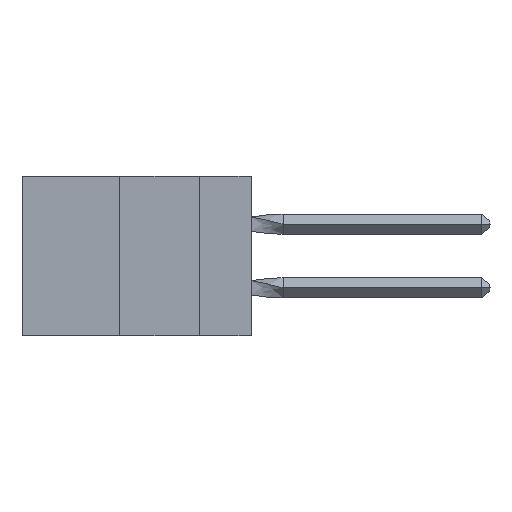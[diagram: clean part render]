
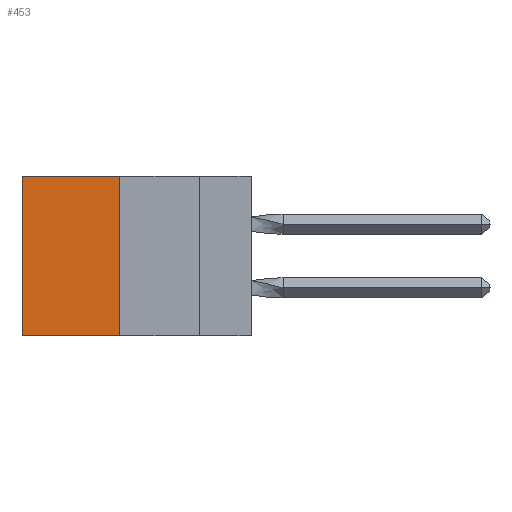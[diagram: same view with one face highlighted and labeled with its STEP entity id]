
A CAD part, left-side view. The second image highlights one B-rep face of the part: STEP entity #453.
In plain terms, the highlighted planar face has unit normal (-1, 0, 0).
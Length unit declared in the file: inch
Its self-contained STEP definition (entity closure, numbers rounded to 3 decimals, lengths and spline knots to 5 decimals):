
#450 = EDGE_CURVE ( 'NONE', #2430, #16674, #26273, .T. ) ;
#453 = ADVANCED_FACE ( 'NONE', ( #7988 ), #14842, .F. ) ;
#598 = EDGE_CURVE ( 'NONE', #6258, #15881, #14458, .T. ) ;
#779 = LINE ( 'NONE', #3295, #23104 ) ;
#1142 = CARTESIAN_POINT ( 'NONE',  ( 0.305, 0.72, 0. ) ) ;
#2425 = DIRECTION ( 'NONE',  ( 0., 0., -1. ) ) ;
#2430 = VERTEX_POINT ( 'NONE', #19436 ) ;
#3295 = CARTESIAN_POINT ( 'NONE',  ( 0.305, 0.413, 0. ) ) ;
#5922 = ORIENTED_EDGE ( 'NONE', *, *, #598, .T. ) ;
#6258 = VERTEX_POINT ( 'NONE', #1142 ) ;
#6452 = EDGE_CURVE ( 'NONE', #16674, #15881, #7986, .T. ) ;
#6819 = CARTESIAN_POINT ( 'NONE',  ( 0.305, 0.72, -0.5 ) ) ;
#7986 = LINE ( 'NONE', #21647, #10041 ) ;
#7988 = FACE_OUTER_BOUND ( 'NONE', #17832, .T. ) ;
#8492 = ORIENTED_EDGE ( 'NONE', *, *, #6452, .F. ) ;
#8943 = DIRECTION ( 'NONE',  ( 0., 1., 0. ) ) ;
#10041 = VECTOR ( 'NONE', #8943, 39.37008 ) ;
#10496 = CARTESIAN_POINT ( 'NONE',  ( 0.305, 0.413, -0.5 ) ) ;
#10562 = ORIENTED_EDGE ( 'NONE', *, *, #24428, .T. ) ;
#11184 = CARTESIAN_POINT ( 'NONE',  ( 0.305, 0.72, -0.5 ) ) ;
#12481 = DIRECTION ( 'NONE',  ( 0., 0., -1. ) ) ;
#14458 = LINE ( 'NONE', #11184, #22874 ) ;
#14842 = PLANE ( 'NONE',  #21778 ) ;
#15881 = VERTEX_POINT ( 'NONE', #6819 ) ;
#16674 = VERTEX_POINT ( 'NONE', #21477 ) ;
#17832 = EDGE_LOOP ( 'NONE', ( #5922, #8492, #26633, #10562 ) ) ;
#19436 = CARTESIAN_POINT ( 'NONE',  ( 0.305, 0.413, 0. ) ) ;
#21124 = CARTESIAN_POINT ( 'NONE',  ( 0.305, 0.413, -0.5 ) ) ;
#21477 = CARTESIAN_POINT ( 'NONE',  ( 0.305, 0.413, -0.5 ) ) ;
#21647 = CARTESIAN_POINT ( 'NONE',  ( 0.305, 0.413, -0.5 ) ) ;
#21778 = AXIS2_PLACEMENT_3D ( 'NONE', #21124, #25761, #12481 ) ;
#22874 = VECTOR ( 'NONE', #2425, 39.37008 ) ;
#23104 = VECTOR ( 'NONE', #26856, 39.37008 ) ;
#24428 = EDGE_CURVE ( 'NONE', #2430, #6258, #779, .T. ) ;
#25761 = DIRECTION ( 'NONE',  ( 1., 0., 0. ) ) ;
#26273 = LINE ( 'NONE', #10496, #26944 ) ;
#26633 = ORIENTED_EDGE ( 'NONE', *, *, #450, .F. ) ;
#26856 = DIRECTION ( 'NONE',  ( 0., 1., 0. ) ) ;
#26944 = VECTOR ( 'NONE', #27945, 39.37008 ) ;
#27945 = DIRECTION ( 'NONE',  ( 0., 0., -1. ) ) ;
